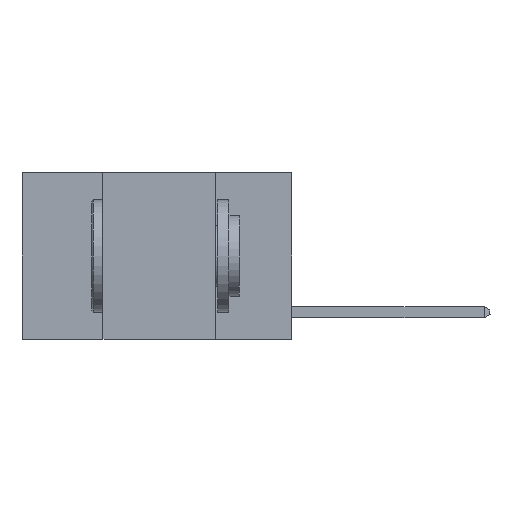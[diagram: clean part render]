
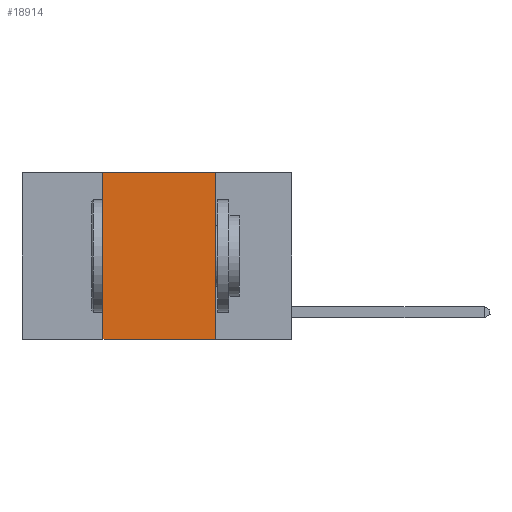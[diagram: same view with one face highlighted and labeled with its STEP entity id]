
A CAD part, left-side view. The second image highlights one B-rep face of the part: STEP entity #18914.
In plain terms, the highlighted planar face has unit normal (-1, 0, 0).
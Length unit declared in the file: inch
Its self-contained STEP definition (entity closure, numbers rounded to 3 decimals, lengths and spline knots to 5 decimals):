
#239 = DIRECTION ( 'NONE',  ( 0., -1., 0. ) ) ;
#435 = VECTOR ( 'NONE', #14112, 39.37008 ) ;
#1221 = CARTESIAN_POINT ( 'NONE',  ( 0., 0.17, 0. ) ) ;
#1509 = CARTESIAN_POINT ( 'NONE',  ( 0., 0.6, 0. ) ) ;
#2951 = ORIENTED_EDGE ( 'NONE', *, *, #23820, .F. ) ;
#3606 = DIRECTION ( 'NONE',  ( 0., -1., 0. ) ) ;
#4004 = LINE ( 'NONE', #1509, #11859 ) ;
#5042 = EDGE_CURVE ( 'NONE', #15297, #19694, #22073, .T. ) ;
#5913 = VECTOR ( 'NONE', #10079, 39.37008 ) ;
#7343 = CARTESIAN_POINT ( 'NONE',  ( 0., 0.17, -0.37 ) ) ;
#7352 = CARTESIAN_POINT ( 'NONE',  ( 0., 0.42, 0. ) ) ;
#9398 = FACE_OUTER_BOUND ( 'NONE', #21355, .T. ) ;
#9929 = LINE ( 'NONE', #21784, #435 ) ;
#9936 = VERTEX_POINT ( 'NONE', #7343 ) ;
#10079 = DIRECTION ( 'NONE',  ( 0., 0., 1. ) ) ;
#10604 = CARTESIAN_POINT ( 'NONE',  ( 0., 0.6, -0.37 ) ) ;
#11635 = CARTESIAN_POINT ( 'NONE',  ( 0., 0.6, 0. ) ) ;
#11859 = VECTOR ( 'NONE', #3606, 39.37008 ) ;
#13268 = VERTEX_POINT ( 'NONE', #1221 ) ;
#14112 = DIRECTION ( 'NONE',  ( 0., 0., -1. ) ) ;
#15297 = VERTEX_POINT ( 'NONE', #16243 ) ;
#16243 = CARTESIAN_POINT ( 'NONE',  ( 0., 0.42, -0.37 ) ) ;
#16409 = VECTOR ( 'NONE', #239, 39.37008 ) ;
#17509 = DIRECTION ( 'NONE',  ( 0., 0., -1. ) ) ;
#18115 = ORIENTED_EDGE ( 'NONE', *, *, #19049, .F. ) ;
#18914 = ADVANCED_FACE ( 'NONE', ( #9398 ), #23239, .F. ) ;
#19049 = EDGE_CURVE ( 'NONE', #13268, #9936, #9929, .T. ) ;
#19694 = VERTEX_POINT ( 'NONE', #7352 ) ;
#19994 = CARTESIAN_POINT ( 'NONE',  ( 0., 0.42, 0. ) ) ;
#20510 = EDGE_CURVE ( 'NONE', #15297, #9936, #24177, .T. ) ;
#21355 = EDGE_LOOP ( 'NONE', ( #18115, #2951, #21616, #21625 ) ) ;
#21616 = ORIENTED_EDGE ( 'NONE', *, *, #5042, .F. ) ;
#21625 = ORIENTED_EDGE ( 'NONE', *, *, #20510, .T. ) ;
#21784 = CARTESIAN_POINT ( 'NONE',  ( 0., 0.17, 0. ) ) ;
#22073 = LINE ( 'NONE', #19994, #5913 ) ;
#22161 = AXIS2_PLACEMENT_3D ( 'NONE', #11635, #23098, #17509 ) ;
#23098 = DIRECTION ( 'NONE',  ( 1., 0., 0. ) ) ;
#23239 = PLANE ( 'NONE',  #22161 ) ;
#23820 = EDGE_CURVE ( 'NONE', #19694, #13268, #4004, .T. ) ;
#24177 = LINE ( 'NONE', #10604, #16409 ) ;
